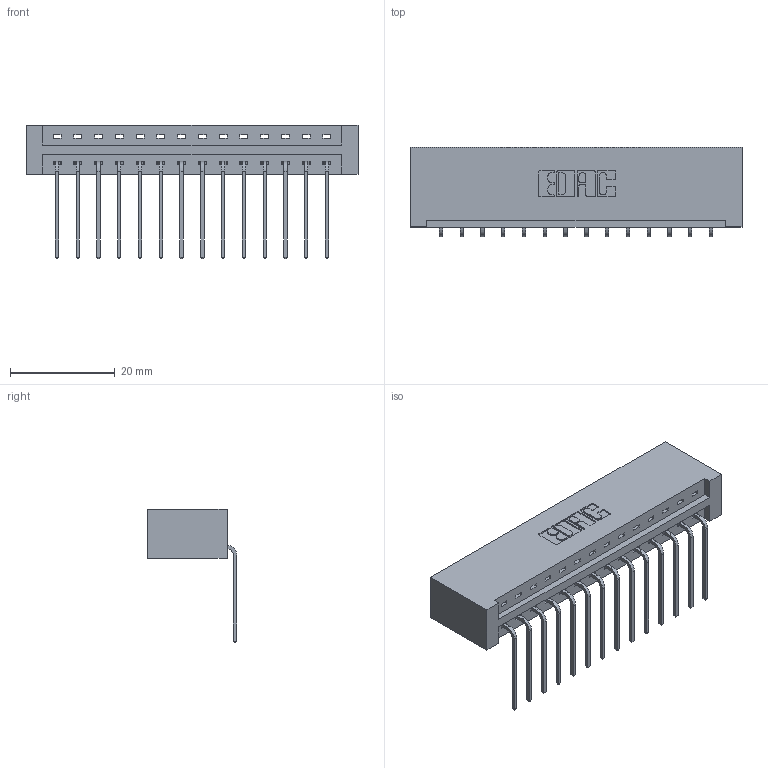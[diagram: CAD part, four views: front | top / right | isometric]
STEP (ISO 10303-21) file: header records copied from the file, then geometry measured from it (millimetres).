
FILE_DESCRIPTION (( 'STEP AP203' ), '1' );
FILE_NAME ('387-014-559-101.STEP', '2018-09-11T06:17:18', ( '' ), ( '' ), 'SwSTEP 2.0', 'SolidWorks 2016', '' );
FILE_SCHEMA (( 'CONFIG_CONTROL_DESIGN' ));
Length unit declared in the file: inch
Products named in the file (3): 337 Part_No Mounting Lugs; 345-292-001_558 559 Tail - 1; 387-014-559-101
Assembly tree (15 placements, depth 2):
  387-014-559-101
    337 Part_No Mounting Lugs
    345-292-001_558 559 Tail - 1  x14
Bounding box: 63.35 x 17.09 x 25.53 mm (x, y, z)
Volume: 7018.9 mm3; surface area: 7365.6 mm2
Topology: 15 solids, 15 shells, 1002 faces, 3003 edges, 1982 vertices
Faces by surface type: plane 738, cylinder 264
Entity records: 13835 total; most frequent: CARTESIAN_POINT 2416, ORIENTED_EDGE 2366, DIRECTION 2083, EDGE_CURVE 1183, VECTOR 1063, LINE 1063, VERTEX_POINT 786, AXIS2_PLACEMENT_3D 510
